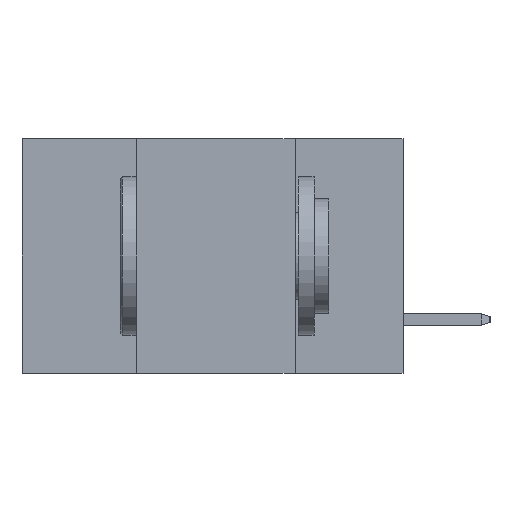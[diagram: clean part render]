
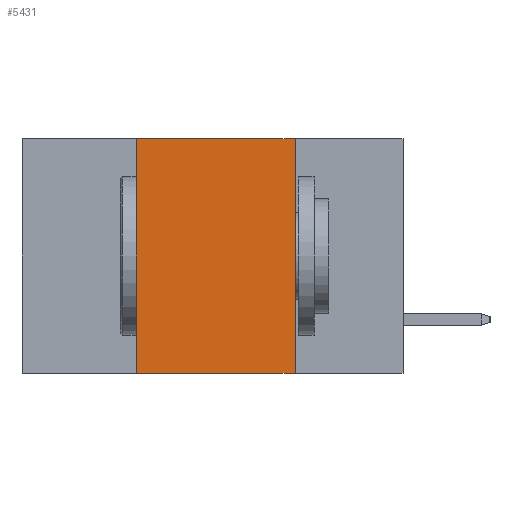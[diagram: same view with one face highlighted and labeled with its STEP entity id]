
A CAD part, left-side view. The second image highlights one B-rep face of the part: STEP entity #5431.
In plain terms, the highlighted planar face has unit normal (-1, 0, 0).
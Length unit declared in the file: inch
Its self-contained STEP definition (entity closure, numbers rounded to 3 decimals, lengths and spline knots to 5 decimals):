
#83 = VERTEX_POINT ( 'NONE', #382 ) ;
#84 = ORIENTED_EDGE ( 'NONE', *, *, #10166, .F. ) ;
#382 = CARTESIAN_POINT ( 'NONE',  ( 0., 0.42, -0.37 ) ) ;
#864 = ORIENTED_EDGE ( 'NONE', *, *, #9176, .F. ) ;
#1045 = LINE ( 'NONE', #6582, #7512 ) ;
#1498 = DIRECTION ( 'NONE',  ( 0., 0., 1. ) ) ;
#1686 = EDGE_LOOP ( 'NONE', ( #864, #84, #4099, #9273 ) ) ;
#1711 = VECTOR ( 'NONE', #4050, 39.37008 ) ;
#1818 = CARTESIAN_POINT ( 'NONE',  ( 0., 0.17, -0.37 ) ) ;
#2148 = LINE ( 'NONE', #7853, #1711 ) ;
#2740 = CARTESIAN_POINT ( 'NONE',  ( 0., 0.17, 0. ) ) ;
#2867 = CARTESIAN_POINT ( 'NONE',  ( 0., 0.6, 0. ) ) ;
#3346 = VECTOR ( 'NONE', #1498, 39.37008 ) ;
#3871 = CARTESIAN_POINT ( 'NONE',  ( 0., 0.42, 0. ) ) ;
#4050 = DIRECTION ( 'NONE',  ( 0., -1., 0. ) ) ;
#4099 = ORIENTED_EDGE ( 'NONE', *, *, #8536, .F. ) ;
#4438 = VERTEX_POINT ( 'NONE', #1818 ) ;
#4692 = CARTESIAN_POINT ( 'NONE',  ( 0., 0.6, 0. ) ) ;
#5227 = DIRECTION ( 'NONE',  ( 0., 0., -1. ) ) ;
#5230 = DIRECTION ( 'NONE',  ( 0., 0., -1. ) ) ;
#5368 = LINE ( 'NONE', #3871, #3346 ) ;
#5431 = ADVANCED_FACE ( 'NONE', ( #6802 ), #9965, .F. ) ;
#5591 = VERTEX_POINT ( 'NONE', #10167 ) ;
#5628 = AXIS2_PLACEMENT_3D ( 'NONE', #2867, #6008, #5230 ) ;
#6008 = DIRECTION ( 'NONE',  ( 1., 0., 0. ) ) ;
#6582 = CARTESIAN_POINT ( 'NONE',  ( 0., 0.17, 0. ) ) ;
#6802 = FACE_OUTER_BOUND ( 'NONE', #1686, .T. ) ;
#6857 = VECTOR ( 'NONE', #7865, 39.37008 ) ;
#7512 = VECTOR ( 'NONE', #5227, 39.37008 ) ;
#7613 = LINE ( 'NONE', #4692, #6857 ) ;
#7853 = CARTESIAN_POINT ( 'NONE',  ( 0., 0.6, -0.37 ) ) ;
#7865 = DIRECTION ( 'NONE',  ( 0., -1., 0. ) ) ;
#8304 = VERTEX_POINT ( 'NONE', #2740 ) ;
#8536 = EDGE_CURVE ( 'NONE', #83, #5591, #5368, .T. ) ;
#8901 = EDGE_CURVE ( 'NONE', #83, #4438, #2148, .T. ) ;
#9176 = EDGE_CURVE ( 'NONE', #8304, #4438, #1045, .T. ) ;
#9273 = ORIENTED_EDGE ( 'NONE', *, *, #8901, .T. ) ;
#9965 = PLANE ( 'NONE',  #5628 ) ;
#10166 = EDGE_CURVE ( 'NONE', #5591, #8304, #7613, .T. ) ;
#10167 = CARTESIAN_POINT ( 'NONE',  ( 0., 0.42, 0. ) ) ;
